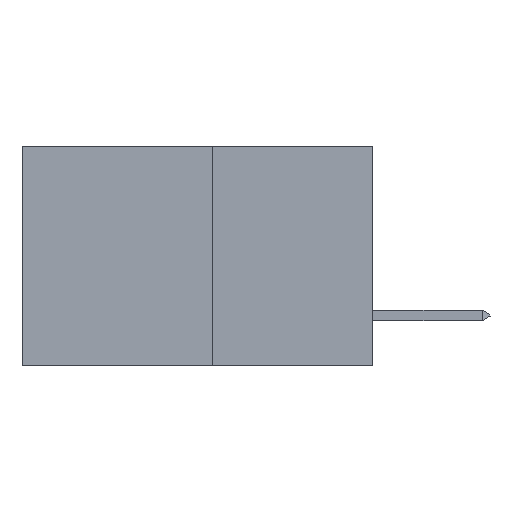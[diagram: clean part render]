
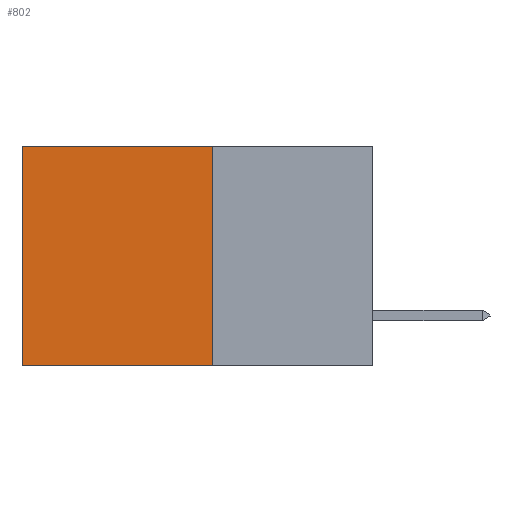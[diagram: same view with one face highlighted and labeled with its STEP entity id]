
A CAD part, left-side view. The second image highlights one B-rep face of the part: STEP entity #802.
In plain terms, the highlighted planar face has unit normal (-1, 0, 0).
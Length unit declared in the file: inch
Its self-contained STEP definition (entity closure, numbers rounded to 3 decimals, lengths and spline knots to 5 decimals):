
#11 = CARTESIAN_POINT ( 'NONE',  ( 0.277, 0.59, -0.37 ) ) ;
#530 = CARTESIAN_POINT ( 'NONE',  ( 0.277, 0.27, -0.37 ) ) ;
#697 = VERTEX_POINT ( 'NONE', #12187 ) ;
#802 = ADVANCED_FACE ( 'NONE', ( #10046 ), #8842, .F. ) ;
#809 = LINE ( 'NONE', #8394, #12638 ) ;
#1646 = DIRECTION ( 'NONE',  ( 0., 0., -1. ) ) ;
#3755 = CARTESIAN_POINT ( 'NONE',  ( 0.277, 0.27, 0. ) ) ;
#4521 = VECTOR ( 'NONE', #8863, 39.37008 ) ;
#4869 = CARTESIAN_POINT ( 'NONE',  ( 0.277, 0.59, -0.37 ) ) ;
#5192 = VECTOR ( 'NONE', #6117, 39.37008 ) ;
#6117 = DIRECTION ( 'NONE',  ( 0., 1., 0. ) ) ;
#6156 = DIRECTION ( 'NONE',  ( 0., 0., -1. ) ) ;
#6561 = AXIS2_PLACEMENT_3D ( 'NONE', #7736, #13952, #6156 ) ;
#7333 = EDGE_CURVE ( 'NONE', #697, #7451, #10375, .T. ) ;
#7451 = VERTEX_POINT ( 'NONE', #4869 ) ;
#7607 = VECTOR ( 'NONE', #13907, 39.37008 ) ;
#7736 = CARTESIAN_POINT ( 'NONE',  ( 0.277, 0.27, -0.37 ) ) ;
#7842 = ORIENTED_EDGE ( 'NONE', *, *, #11406, .F. ) ;
#8394 = CARTESIAN_POINT ( 'NONE',  ( 0.277, 0.27, -0.37 ) ) ;
#8524 = EDGE_CURVE ( 'NONE', #9101, #697, #13599, .T. ) ;
#8842 = PLANE ( 'NONE',  #6561 ) ;
#8863 = DIRECTION ( 'NONE',  ( 0., 0., -1. ) ) ;
#9101 = VERTEX_POINT ( 'NONE', #3755 ) ;
#9234 = EDGE_CURVE ( 'NONE', #10085, #7451, #10490, .T. ) ;
#9726 = ORIENTED_EDGE ( 'NONE', *, *, #8524, .T. ) ;
#9751 = ORIENTED_EDGE ( 'NONE', *, *, #9234, .F. ) ;
#10046 = FACE_OUTER_BOUND ( 'NONE', #12449, .T. ) ;
#10085 = VERTEX_POINT ( 'NONE', #12429 ) ;
#10375 = LINE ( 'NONE', #11, #4521 ) ;
#10490 = LINE ( 'NONE', #530, #7607 ) ;
#11406 = EDGE_CURVE ( 'NONE', #9101, #10085, #809, .T. ) ;
#11560 = CARTESIAN_POINT ( 'NONE',  ( 0.277, 0.27, 0. ) ) ;
#12187 = CARTESIAN_POINT ( 'NONE',  ( 0.277, 0.59, 0. ) ) ;
#12293 = ORIENTED_EDGE ( 'NONE', *, *, #7333, .T. ) ;
#12429 = CARTESIAN_POINT ( 'NONE',  ( 0.277, 0.27, -0.37 ) ) ;
#12449 = EDGE_LOOP ( 'NONE', ( #12293, #9751, #7842, #9726 ) ) ;
#12638 = VECTOR ( 'NONE', #1646, 39.37008 ) ;
#13599 = LINE ( 'NONE', #11560, #5192 ) ;
#13907 = DIRECTION ( 'NONE',  ( 0., 1., 0. ) ) ;
#13952 = DIRECTION ( 'NONE',  ( 1., 0., 0. ) ) ;
